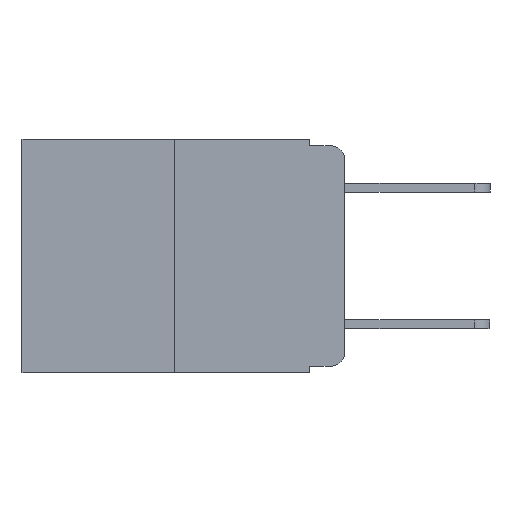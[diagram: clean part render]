
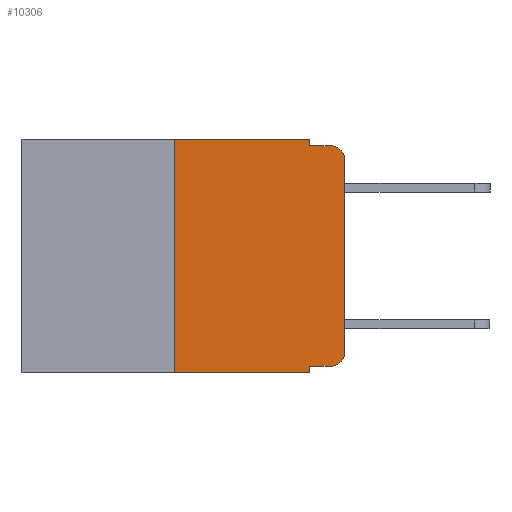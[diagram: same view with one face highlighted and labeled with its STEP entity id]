
A CAD part, left-side view. The second image highlights one B-rep face of the part: STEP entity #10306.
In plain terms, the highlighted planar face has unit normal (-1, 0, 0).
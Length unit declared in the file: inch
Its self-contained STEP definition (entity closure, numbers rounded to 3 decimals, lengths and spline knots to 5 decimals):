
#384 = VERTEX_POINT ( 'NONE', #19843 ) ;
#409 = DIRECTION ( 'NONE',  ( 0., -1., 0. ) ) ;
#532 = LINE ( 'NONE', #15578, #13347 ) ;
#1150 = VERTEX_POINT ( 'NONE', #6144 ) ;
#1421 = DIRECTION ( 'NONE',  ( 0., 0., -1. ) ) ;
#1688 = VERTEX_POINT ( 'NONE', #4283 ) ;
#1799 = DIRECTION ( 'NONE',  ( 0., 0., -1. ) ) ;
#1870 = EDGE_CURVE ( 'NONE', #8293, #20250, #6228, .T. ) ;
#3590 = CARTESIAN_POINT ( 'NONE',  ( 0., 0.02, -0.333 ) ) ;
#4110 = VECTOR ( 'NONE', #409, 39.37008 ) ;
#4283 = CARTESIAN_POINT ( 'NONE',  ( 0., 0., -0.313 ) ) ;
#5010 = LINE ( 'NONE', #18153, #14044 ) ;
#5163 = ORIENTED_EDGE ( 'NONE', *, *, #7610, .T. ) ;
#5343 = EDGE_CURVE ( 'NONE', #20250, #384, #5010, .T. ) ;
#5633 = VERTEX_POINT ( 'NONE', #6527 ) ;
#5705 = ORIENTED_EDGE ( 'NONE', *, *, #6508, .T. ) ;
#5707 = VECTOR ( 'NONE', #13842, 39.37008 ) ;
#5814 = ORIENTED_EDGE ( 'NONE', *, *, #5343, .F. ) ;
#6144 = CARTESIAN_POINT ( 'NONE',  ( 0., 0., -0.03 ) ) ;
#6228 = LINE ( 'NONE', #7368, #5707 ) ;
#6431 = CARTESIAN_POINT ( 'NONE',  ( 0., 0.051, 0. ) ) ;
#6508 = EDGE_CURVE ( 'NONE', #1150, #384, #17181, .T. ) ;
#6527 = CARTESIAN_POINT ( 'NONE',  ( 0., 0.25, -0.343 ) ) ;
#6704 = DIRECTION ( 'NONE',  ( -1., 0., 0. ) ) ;
#7368 = CARTESIAN_POINT ( 'NONE',  ( 0., 0.051, 0. ) ) ;
#7499 = VERTEX_POINT ( 'NONE', #3590 ) ;
#7508 = LINE ( 'NONE', #6431, #19260 ) ;
#7610 = EDGE_CURVE ( 'NONE', #1688, #1150, #13856, .T. ) ;
#7852 = CARTESIAN_POINT ( 'NONE',  ( 0., 0.25, 0. ) ) ;
#7998 = CIRCLE ( 'NONE', #16114, 0.02 ) ;
#8048 = AXIS2_PLACEMENT_3D ( 'NONE', #16067, #6704, #17566 ) ;
#8084 = FACE_OUTER_BOUND ( 'NONE', #12179, .T. ) ;
#8215 = VERTEX_POINT ( 'NONE', #9247 ) ;
#8293 = VERTEX_POINT ( 'NONE', #15542 ) ;
#8957 = DIRECTION ( 'NONE',  ( 0., -1., 0. ) ) ;
#9053 = VERTEX_POINT ( 'NONE', #12774 ) ;
#9200 = VERTEX_POINT ( 'NONE', #16151 ) ;
#9247 = CARTESIAN_POINT ( 'NONE',  ( 0., 0.25, 0. ) ) ;
#9483 = DIRECTION ( 'NONE',  ( 0., 0., 1. ) ) ;
#9708 = VECTOR ( 'NONE', #18044, 39.37008 ) ;
#9727 = VECTOR ( 'NONE', #9483, 39.37008 ) ;
#9876 = PLANE ( 'NONE',  #17802 ) ;
#10087 = EDGE_CURVE ( 'NONE', #8215, #8293, #20452, .T. ) ;
#10306 = ADVANCED_FACE ( 'NONE', ( #8084 ), #9876, .F. ) ;
#10797 = CARTESIAN_POINT ( 'NONE',  ( 0., 0.473, 0. ) ) ;
#11038 = DIRECTION ( 'NONE',  ( 0., -1., 0. ) ) ;
#11469 = DIRECTION ( 'NONE',  ( 1., 0., 0. ) ) ;
#11496 = ORIENTED_EDGE ( 'NONE', *, *, #1870, .F. ) ;
#11766 = DIRECTION ( 'NONE',  ( -1., 0., 0. ) ) ;
#12179 = EDGE_LOOP ( 'NONE', ( #5163, #5705, #5814, #11496, #13137, #13562, #13582, #15956, #16825, #17113 ) ) ;
#12228 = LINE ( 'NONE', #19682, #4110 ) ;
#12774 = CARTESIAN_POINT ( 'NONE',  ( 0., 0.051, -0.343 ) ) ;
#12837 = DIRECTION ( 'NONE',  ( 0., 0., -1. ) ) ;
#13137 = ORIENTED_EDGE ( 'NONE', *, *, #10087, .F. ) ;
#13347 = VECTOR ( 'NONE', #11038, 39.37008 ) ;
#13542 = CARTESIAN_POINT ( 'NONE',  ( 0., 0., 0. ) ) ;
#13562 = ORIENTED_EDGE ( 'NONE', *, *, #20236, .F. ) ;
#13582 = ORIENTED_EDGE ( 'NONE', *, *, #15840, .T. ) ;
#13842 = DIRECTION ( 'NONE',  ( 0., 0., -1. ) ) ;
#13856 = LINE ( 'NONE', #13542, #9708 ) ;
#13884 = DIRECTION ( 'NONE',  ( 0., -1., 0. ) ) ;
#14044 = VECTOR ( 'NONE', #8957, 39.37008 ) ;
#15542 = CARTESIAN_POINT ( 'NONE',  ( 0., 0.051, 0. ) ) ;
#15578 = CARTESIAN_POINT ( 'NONE',  ( 0., 0.051, -0.333 ) ) ;
#15635 = CARTESIAN_POINT ( 'NONE',  ( 0., 0.051, -0.01 ) ) ;
#15840 = EDGE_CURVE ( 'NONE', #5633, #9053, #12228, .T. ) ;
#15956 = ORIENTED_EDGE ( 'NONE', *, *, #19273, .F. ) ;
#16067 = CARTESIAN_POINT ( 'NONE',  ( 0., 0.02, -0.03 ) ) ;
#16113 = VECTOR ( 'NONE', #13884, 39.37008 ) ;
#16114 = AXIS2_PLACEMENT_3D ( 'NONE', #20669, #11766, #1799 ) ;
#16151 = CARTESIAN_POINT ( 'NONE',  ( 0., 0.051, -0.333 ) ) ;
#16322 = EDGE_CURVE ( 'NONE', #7499, #1688, #7998, .T. ) ;
#16825 = ORIENTED_EDGE ( 'NONE', *, *, #17320, .T. ) ;
#17113 = ORIENTED_EDGE ( 'NONE', *, *, #16322, .T. ) ;
#17181 = CIRCLE ( 'NONE', #8048, 0.02 ) ;
#17320 = EDGE_CURVE ( 'NONE', #9200, #7499, #532, .T. ) ;
#17396 = LINE ( 'NONE', #7852, #9727 ) ;
#17566 = DIRECTION ( 'NONE',  ( 0., 0., -1. ) ) ;
#17802 = AXIS2_PLACEMENT_3D ( 'NONE', #18958, #11469, #1421 ) ;
#18044 = DIRECTION ( 'NONE',  ( 0., 0., 1. ) ) ;
#18153 = CARTESIAN_POINT ( 'NONE',  ( 0., 0.051, -0.01 ) ) ;
#18958 = CARTESIAN_POINT ( 'NONE',  ( 0., 0.473, 0. ) ) ;
#19260 = VECTOR ( 'NONE', #12837, 39.37008 ) ;
#19273 = EDGE_CURVE ( 'NONE', #9200, #9053, #7508, .T. ) ;
#19682 = CARTESIAN_POINT ( 'NONE',  ( 0., 0.473, -0.343 ) ) ;
#19843 = CARTESIAN_POINT ( 'NONE',  ( 0., 0.02, -0.01 ) ) ;
#20236 = EDGE_CURVE ( 'NONE', #5633, #8215, #17396, .T. ) ;
#20250 = VERTEX_POINT ( 'NONE', #15635 ) ;
#20452 = LINE ( 'NONE', #10797, #16113 ) ;
#20669 = CARTESIAN_POINT ( 'NONE',  ( 0., 0.02, -0.313 ) ) ;
